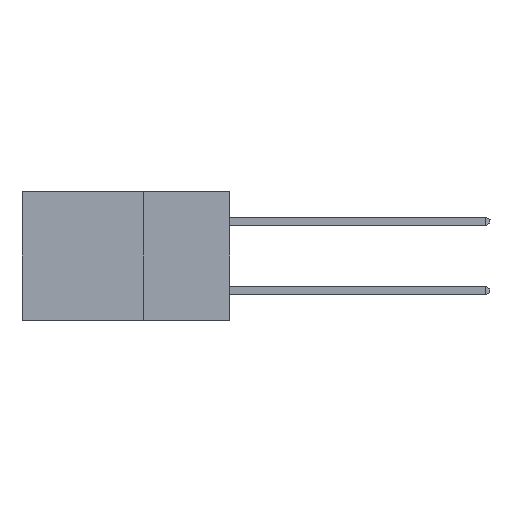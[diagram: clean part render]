
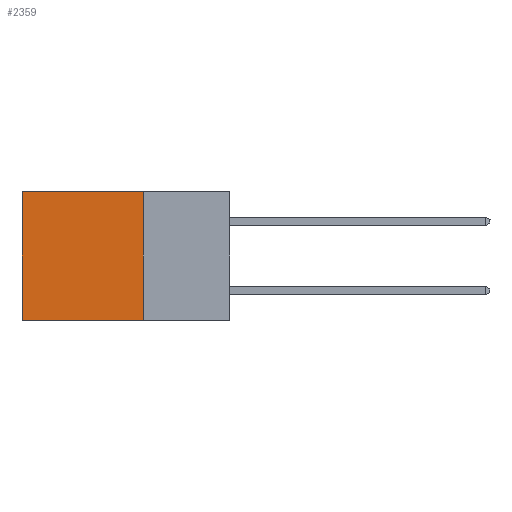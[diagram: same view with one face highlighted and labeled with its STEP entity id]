
A CAD part, left-side view. The second image highlights one B-rep face of the part: STEP entity #2359.
In plain terms, the highlighted planar face has unit normal (-1, 0, 0).
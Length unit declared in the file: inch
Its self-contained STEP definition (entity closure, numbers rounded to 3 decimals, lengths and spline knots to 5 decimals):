
#10 = EDGE_CURVE ( 'NONE', #2550, #9903, #925, .T. ) ;
#199 = ORIENTED_EDGE ( 'NONE', *, *, #10693, .F. ) ;
#337 = EDGE_LOOP ( 'NONE', ( #11445, #7107, #199, #5098 ) ) ;
#472 = FACE_OUTER_BOUND ( 'NONE', #337, .T. ) ;
#863 = CARTESIAN_POINT ( 'NONE',  ( 0.298, 0.6, 0. ) ) ;
#925 = LINE ( 'NONE', #2350, #1388 ) ;
#1056 = VERTEX_POINT ( 'NONE', #863 ) ;
#1101 = VERTEX_POINT ( 'NONE', #5868 ) ;
#1388 = VECTOR ( 'NONE', #3206, 39.37008 ) ;
#1502 = LINE ( 'NONE', #9731, #4845 ) ;
#1928 = CARTESIAN_POINT ( 'NONE',  ( 0.298, 0.25, -0.37 ) ) ;
#2350 = CARTESIAN_POINT ( 'NONE',  ( 0.298, 0.25, -0.37 ) ) ;
#2359 = ADVANCED_FACE ( 'NONE', ( #472 ), #5594, .F. ) ;
#2550 = VERTEX_POINT ( 'NONE', #1928 ) ;
#3037 = DIRECTION ( 'NONE',  ( 0., 1., 0. ) ) ;
#3206 = DIRECTION ( 'NONE',  ( 0., 1., 0. ) ) ;
#3535 = CARTESIAN_POINT ( 'NONE',  ( 0.298, 0.25, 0. ) ) ;
#3665 = AXIS2_PLACEMENT_3D ( 'NONE', #3535, #12211, #4620 ) ;
#4442 = CARTESIAN_POINT ( 'NONE',  ( 0.298, 0.25, 0. ) ) ;
#4620 = DIRECTION ( 'NONE',  ( 0., 0., -1. ) ) ;
#4845 = VECTOR ( 'NONE', #3037, 39.37008 ) ;
#5098 = ORIENTED_EDGE ( 'NONE', *, *, #12193, .T. ) ;
#5594 = PLANE ( 'NONE',  #3665 ) ;
#5678 = DIRECTION ( 'NONE',  ( 0., 0., -1. ) ) ;
#5868 = CARTESIAN_POINT ( 'NONE',  ( 0.298, 0.25, 0. ) ) ;
#6457 = VECTOR ( 'NONE', #11201, 39.37008 ) ;
#7040 = VECTOR ( 'NONE', #5678, 39.37008 ) ;
#7107 = ORIENTED_EDGE ( 'NONE', *, *, #10, .F. ) ;
#7807 = LINE ( 'NONE', #4442, #6457 ) ;
#8526 = CARTESIAN_POINT ( 'NONE',  ( 0.298, 0.6, 0. ) ) ;
#9731 = CARTESIAN_POINT ( 'NONE',  ( 0.298, 0.25, 0. ) ) ;
#9903 = VERTEX_POINT ( 'NONE', #12522 ) ;
#10397 = LINE ( 'NONE', #8526, #7040 ) ;
#10693 = EDGE_CURVE ( 'NONE', #1101, #2550, #7807, .T. ) ;
#10939 = EDGE_CURVE ( 'NONE', #1056, #9903, #10397, .T. ) ;
#11201 = DIRECTION ( 'NONE',  ( 0., 0., -1. ) ) ;
#11445 = ORIENTED_EDGE ( 'NONE', *, *, #10939, .T. ) ;
#12193 = EDGE_CURVE ( 'NONE', #1101, #1056, #1502, .T. ) ;
#12211 = DIRECTION ( 'NONE',  ( 1., 0., 0. ) ) ;
#12522 = CARTESIAN_POINT ( 'NONE',  ( 0.298, 0.6, -0.37 ) ) ;
